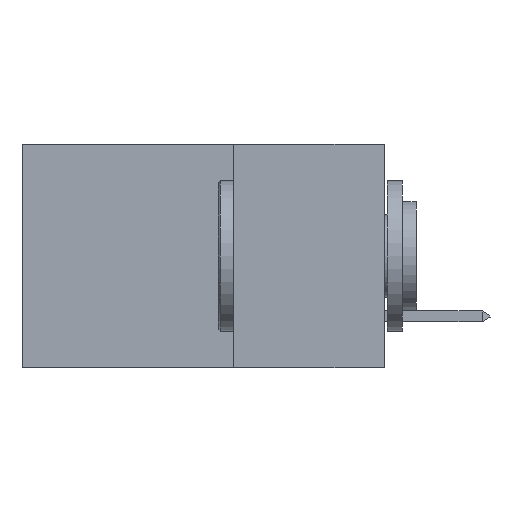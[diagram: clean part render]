
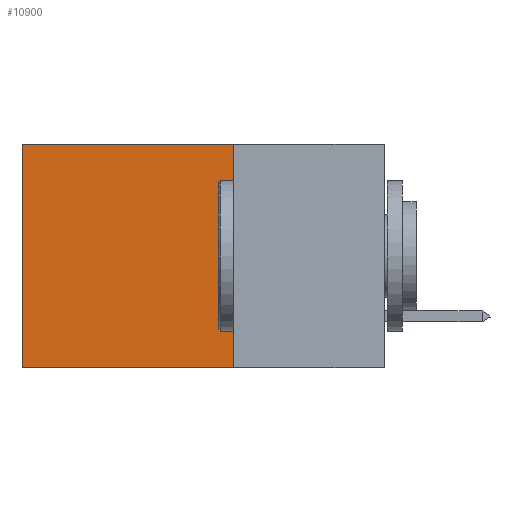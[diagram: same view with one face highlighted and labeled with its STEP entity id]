
A CAD part, left-side view. The second image highlights one B-rep face of the part: STEP entity #10900.
In plain terms, the highlighted planar face has unit normal (-1, 0, 0).
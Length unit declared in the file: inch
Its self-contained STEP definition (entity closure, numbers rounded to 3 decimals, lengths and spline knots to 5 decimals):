
#231 = EDGE_LOOP ( 'NONE', ( #5257, #21375, #17084, #25811 ) ) ;
#2123 = CARTESIAN_POINT ( 'NONE',  ( 0.2875, 0.25, 0. ) ) ;
#2829 = CARTESIAN_POINT ( 'NONE',  ( 0.2875, 0.6, -0.37 ) ) ;
#2861 = CARTESIAN_POINT ( 'NONE',  ( 0.2875, 0.25, 0. ) ) ;
#3217 = AXIS2_PLACEMENT_3D ( 'NONE', #22409, #34392, #16587 ) ;
#3444 = LINE ( 'NONE', #34086, #26648 ) ;
#4106 = VERTEX_POINT ( 'NONE', #6343 ) ;
#5257 = ORIENTED_EDGE ( 'NONE', *, *, #11588, .T. ) ;
#6343 = CARTESIAN_POINT ( 'NONE',  ( 0.2875, 0.25, 0. ) ) ;
#8426 = VERTEX_POINT ( 'NONE', #13598 ) ;
#10609 = PLANE ( 'NONE',  #3217 ) ;
#10900 = ADVANCED_FACE ( 'NONE', ( #28792 ), #10609, .F. ) ;
#11588 = EDGE_CURVE ( 'NONE', #12754, #34252, #27522, .T. ) ;
#12402 = DIRECTION ( 'NONE',  ( 0., 0., -1. ) ) ;
#12754 = VERTEX_POINT ( 'NONE', #16865 ) ;
#12864 = VECTOR ( 'NONE', #32464, 39.37008 ) ;
#13598 = CARTESIAN_POINT ( 'NONE',  ( 0.2875, 0.25, -0.37 ) ) ;
#16285 = DIRECTION ( 'NONE',  ( 0., 1., 0. ) ) ;
#16587 = DIRECTION ( 'NONE',  ( 0., 0., -1. ) ) ;
#16865 = CARTESIAN_POINT ( 'NONE',  ( 0.2875, 0.6, 0. ) ) ;
#17084 = ORIENTED_EDGE ( 'NONE', *, *, #29222, .F. ) ;
#18895 = LINE ( 'NONE', #2861, #12864 ) ;
#21375 = ORIENTED_EDGE ( 'NONE', *, *, #27920, .F. ) ;
#21598 = CARTESIAN_POINT ( 'NONE',  ( 0.2875, 0.6, 0. ) ) ;
#22409 = CARTESIAN_POINT ( 'NONE',  ( 0.2875, 0.25, 0. ) ) ;
#25811 = ORIENTED_EDGE ( 'NONE', *, *, #32461, .T. ) ;
#25892 = DIRECTION ( 'NONE',  ( 0., 0., -1. ) ) ;
#26648 = VECTOR ( 'NONE', #16285, 39.37008 ) ;
#27522 = LINE ( 'NONE', #21598, #28001 ) ;
#27920 = EDGE_CURVE ( 'NONE', #8426, #34252, #3444, .T. ) ;
#28001 = VECTOR ( 'NONE', #12402, 39.37008 ) ;
#28792 = FACE_OUTER_BOUND ( 'NONE', #231, .T. ) ;
#29222 = EDGE_CURVE ( 'NONE', #4106, #8426, #33005, .T. ) ;
#32461 = EDGE_CURVE ( 'NONE', #4106, #12754, #18895, .T. ) ;
#32464 = DIRECTION ( 'NONE',  ( 0., 1., 0. ) ) ;
#33005 = LINE ( 'NONE', #2123, #34457 ) ;
#34086 = CARTESIAN_POINT ( 'NONE',  ( 0.2875, 0.25, -0.37 ) ) ;
#34252 = VERTEX_POINT ( 'NONE', #2829 ) ;
#34392 = DIRECTION ( 'NONE',  ( 1., 0., 0. ) ) ;
#34457 = VECTOR ( 'NONE', #25892, 39.37008 ) ;
